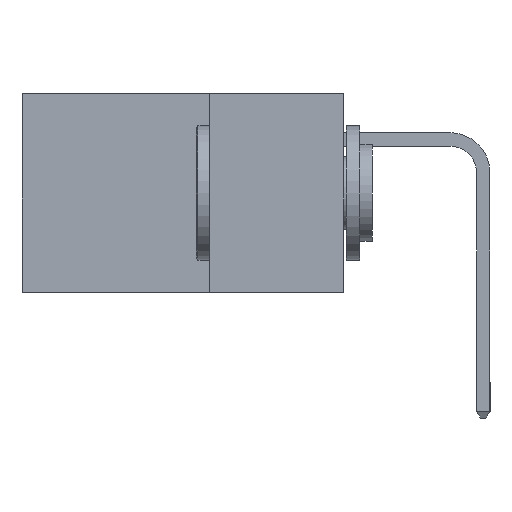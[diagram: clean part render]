
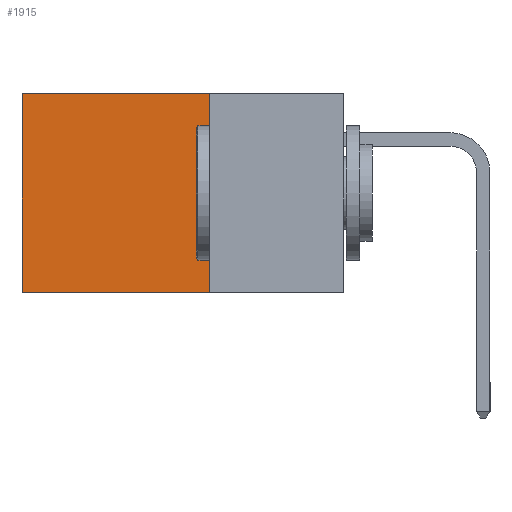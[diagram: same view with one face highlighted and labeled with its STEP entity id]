
A CAD part, left-side view. The second image highlights one B-rep face of the part: STEP entity #1915.
In plain terms, the highlighted planar face has unit normal (-1, 0, 0).
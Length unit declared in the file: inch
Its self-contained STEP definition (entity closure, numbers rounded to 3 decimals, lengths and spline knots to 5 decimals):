
#448 = ORIENTED_EDGE ( 'NONE', *, *, #7107, .T. ) ;
#1568 = VERTEX_POINT ( 'NONE', #3393 ) ;
#1651 = DIRECTION ( 'NONE',  ( 0., 0., -1. ) ) ;
#1823 = ORIENTED_EDGE ( 'NONE', *, *, #15631, .F. ) ;
#1915 = ADVANCED_FACE ( 'NONE', ( #4112 ), #2327, .F. ) ;
#1964 = CARTESIAN_POINT ( 'NONE',  ( 0.298, 0.6, -0.37 ) ) ;
#2237 = LINE ( 'NONE', #2273, #15167 ) ;
#2273 = CARTESIAN_POINT ( 'NONE',  ( 0.298, 0.25, 0. ) ) ;
#2327 = PLANE ( 'NONE',  #14995 ) ;
#2584 = CARTESIAN_POINT ( 'NONE',  ( 0.298, 0.25, -0.37 ) ) ;
#3188 = CARTESIAN_POINT ( 'NONE',  ( 0.298, 0.25, 0. ) ) ;
#3393 = CARTESIAN_POINT ( 'NONE',  ( 0.298, 0.6, 0. ) ) ;
#3748 = DIRECTION ( 'NONE',  ( 1., 0., 0. ) ) ;
#3773 = CARTESIAN_POINT ( 'NONE',  ( 0.298, 0.25, 0. ) ) ;
#4112 = FACE_OUTER_BOUND ( 'NONE', #9593, .T. ) ;
#4542 = DIRECTION ( 'NONE',  ( 0., 0., -1. ) ) ;
#4816 = VERTEX_POINT ( 'NONE', #16094 ) ;
#5094 = VECTOR ( 'NONE', #10858, 39.37008 ) ;
#5147 = EDGE_CURVE ( 'NONE', #4816, #7676, #6787, .T. ) ;
#5199 = VECTOR ( 'NONE', #4542, 39.37008 ) ;
#6351 = CARTESIAN_POINT ( 'NONE',  ( 0.298, 0.25, 0. ) ) ;
#6370 = VECTOR ( 'NONE', #17107, 39.37008 ) ;
#6529 = VERTEX_POINT ( 'NONE', #6351 ) ;
#6787 = LINE ( 'NONE', #2584, #6370 ) ;
#7107 = EDGE_CURVE ( 'NONE', #1568, #7676, #15668, .T. ) ;
#7676 = VERTEX_POINT ( 'NONE', #1964 ) ;
#9593 = EDGE_LOOP ( 'NONE', ( #448, #14993, #1823, #16502 ) ) ;
#10858 = DIRECTION ( 'NONE',  ( 0., 0., -1. ) ) ;
#10909 = CARTESIAN_POINT ( 'NONE',  ( 0.298, 0.6, 0. ) ) ;
#13882 = DIRECTION ( 'NONE',  ( 0., 1., 0. ) ) ;
#14993 = ORIENTED_EDGE ( 'NONE', *, *, #5147, .F. ) ;
#14995 = AXIS2_PLACEMENT_3D ( 'NONE', #3773, #3748, #1651 ) ;
#15167 = VECTOR ( 'NONE', #13882, 39.37008 ) ;
#15631 = EDGE_CURVE ( 'NONE', #6529, #4816, #15764, .T. ) ;
#15668 = LINE ( 'NONE', #10909, #5094 ) ;
#15764 = LINE ( 'NONE', #3188, #5199 ) ;
#15857 = EDGE_CURVE ( 'NONE', #6529, #1568, #2237, .T. ) ;
#16094 = CARTESIAN_POINT ( 'NONE',  ( 0.298, 0.25, -0.37 ) ) ;
#16502 = ORIENTED_EDGE ( 'NONE', *, *, #15857, .T. ) ;
#17107 = DIRECTION ( 'NONE',  ( 0., 1., 0. ) ) ;
